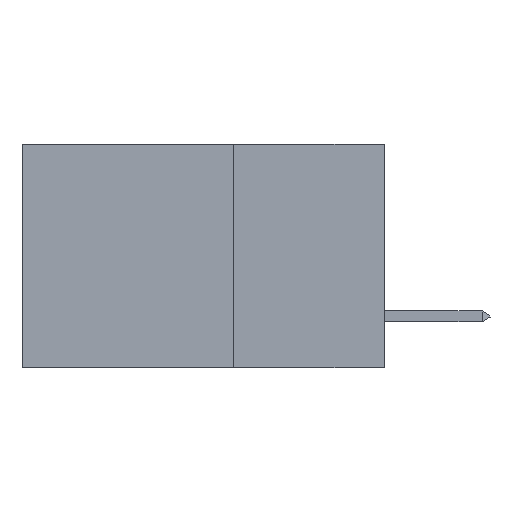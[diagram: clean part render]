
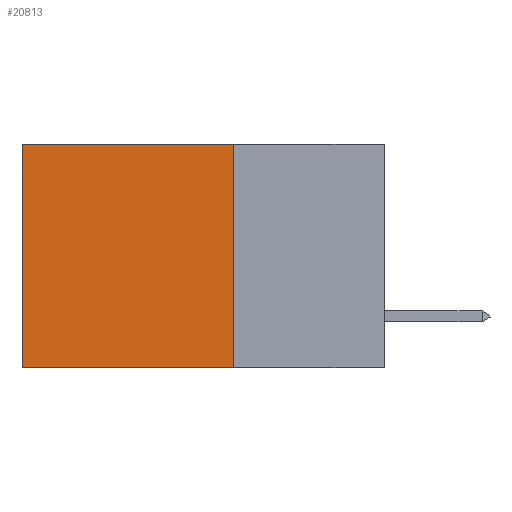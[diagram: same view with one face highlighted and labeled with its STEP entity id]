
A CAD part, left-side view. The second image highlights one B-rep face of the part: STEP entity #20813.
In plain terms, the highlighted planar face has unit normal (-1, 0, 0).
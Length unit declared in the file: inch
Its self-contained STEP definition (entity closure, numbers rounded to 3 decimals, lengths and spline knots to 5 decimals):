
#304 = VECTOR ( 'NONE', #3582, 39.37008 ) ;
#1223 = CARTESIAN_POINT ( 'NONE',  ( 0.2875, 0.25, 0. ) ) ;
#3483 = PLANE ( 'NONE',  #22331 ) ;
#3582 = DIRECTION ( 'NONE',  ( 0., 1., 0. ) ) ;
#3692 = EDGE_CURVE ( 'NONE', #4129, #5703, #4558, .T. ) ;
#4129 = VERTEX_POINT ( 'NONE', #1223 ) ;
#4244 = CARTESIAN_POINT ( 'NONE',  ( 0.2875, 0.25, 0. ) ) ;
#4558 = LINE ( 'NONE', #4244, #11618 ) ;
#4600 = CARTESIAN_POINT ( 'NONE',  ( 0.2875, 0.25, -0.37 ) ) ;
#4941 = LINE ( 'NONE', #22353, #21987 ) ;
#5085 = ORIENTED_EDGE ( 'NONE', *, *, #19456, .T. ) ;
#5285 = CARTESIAN_POINT ( 'NONE',  ( 0.2875, 0.25, 0. ) ) ;
#5321 = LINE ( 'NONE', #18506, #304 ) ;
#5703 = VERTEX_POINT ( 'NONE', #4600 ) ;
#6708 = CARTESIAN_POINT ( 'NONE',  ( 0.2875, 0.6, 0. ) ) ;
#7980 = DIRECTION ( 'NONE',  ( 0., 1., 0. ) ) ;
#8908 = ORIENTED_EDGE ( 'NONE', *, *, #11991, .T. ) ;
#9760 = ORIENTED_EDGE ( 'NONE', *, *, #20441, .F. ) ;
#9898 = FACE_OUTER_BOUND ( 'NONE', #19434, .T. ) ;
#10208 = VECTOR ( 'NONE', #7980, 39.37008 ) ;
#11618 = VECTOR ( 'NONE', #17619, 39.37008 ) ;
#11991 = EDGE_CURVE ( 'NONE', #12781, #15566, #4941, .T. ) ;
#12781 = VERTEX_POINT ( 'NONE', #6708 ) ;
#12888 = DIRECTION ( 'NONE',  ( 0., 0., -1. ) ) ;
#13598 = CARTESIAN_POINT ( 'NONE',  ( 0.2875, 0.25, -0.37 ) ) ;
#15114 = CARTESIAN_POINT ( 'NONE',  ( 0.2875, 0.6, -0.37 ) ) ;
#15566 = VERTEX_POINT ( 'NONE', #15114 ) ;
#16589 = DIRECTION ( 'NONE',  ( 0., 0., -1. ) ) ;
#17619 = DIRECTION ( 'NONE',  ( 0., 0., -1. ) ) ;
#18506 = CARTESIAN_POINT ( 'NONE',  ( 0.2875, 0.25, 0. ) ) ;
#19362 = LINE ( 'NONE', #13598, #10208 ) ;
#19434 = EDGE_LOOP ( 'NONE', ( #8908, #9760, #21541, #5085 ) ) ;
#19456 = EDGE_CURVE ( 'NONE', #4129, #12781, #5321, .T. ) ;
#20441 = EDGE_CURVE ( 'NONE', #5703, #15566, #19362, .T. ) ;
#20813 = ADVANCED_FACE ( 'NONE', ( #9898 ), #3483, .F. ) ;
#21541 = ORIENTED_EDGE ( 'NONE', *, *, #3692, .F. ) ;
#21987 = VECTOR ( 'NONE', #12888, 39.37008 ) ;
#22331 = AXIS2_PLACEMENT_3D ( 'NONE', #5285, #22424, #16589 ) ;
#22353 = CARTESIAN_POINT ( 'NONE',  ( 0.2875, 0.6, 0. ) ) ;
#22424 = DIRECTION ( 'NONE',  ( 1., 0., 0. ) ) ;
